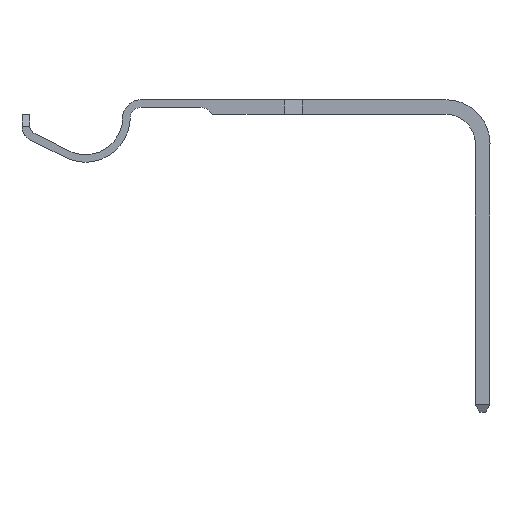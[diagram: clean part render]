
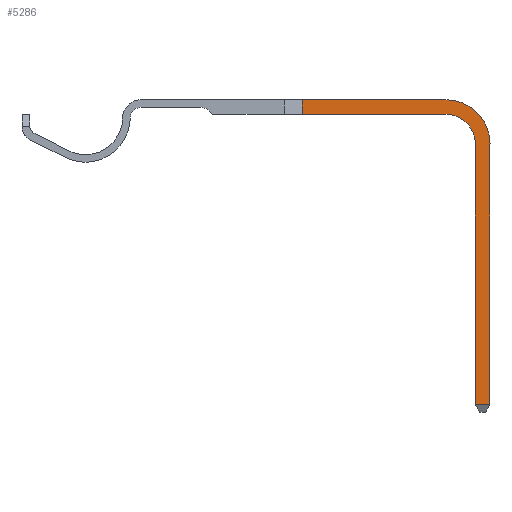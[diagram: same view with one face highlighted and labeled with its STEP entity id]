
A CAD part, left-side view. The second image highlights one B-rep face of the part: STEP entity #5286.
In plain terms, the highlighted face is planar.
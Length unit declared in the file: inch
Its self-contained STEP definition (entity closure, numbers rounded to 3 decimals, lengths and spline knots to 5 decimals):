
#418 = EDGE_CURVE ( 'NONE', #6218, #4069, #11643, .T. ) ;
#1639 = CARTESIAN_POINT ( 'NONE',  ( 0.85571, 0.0375, -0.0125 ) ) ;
#1671 = VECTOR ( 'NONE', #4748, 39.37008 ) ;
#1710 = CARTESIAN_POINT ( 'NONE',  ( 0.61115, 0.0375, -0.0125 ) ) ;
#2480 = VERTEX_POINT ( 'NONE', #5205 ) ;
#2566 = EDGE_LOOP ( 'NONE', ( #3363, #9571, #14567, #13523, #6890, #12255, #6935, #12614 ) ) ;
#2777 = CARTESIAN_POINT ( 'NONE',  ( 0.58021, 0.0125, -0.0125 ) ) ;
#2914 = CARTESIAN_POINT ( 'NONE',  ( 0.85571, 0.0875, -0.0125 ) ) ;
#2934 = DIRECTION ( 'NONE',  ( 0., 1., 0. ) ) ;
#3066 = VECTOR ( 'NONE', #7339, 39.37008 ) ;
#3363 = ORIENTED_EDGE ( 'NONE', *, *, #6491, .T. ) ;
#3424 = LINE ( 'NONE', #2777, #3066 ) ;
#3797 = EDGE_CURVE ( 'NONE', #11314, #6218, #3424, .T. ) ;
#4069 = VERTEX_POINT ( 'NONE', #1710 ) ;
#4230 = EDGE_CURVE ( 'NONE', #9827, #13113, #6945, .T. ) ;
#4748 = DIRECTION ( 'NONE',  ( 0., 1., 0. ) ) ;
#4835 = CARTESIAN_POINT ( 'NONE',  ( 0.93071, 0.532, -0.0125 ) ) ;
#5205 = CARTESIAN_POINT ( 'NONE',  ( 0.93071, 0.0875, -0.0125 ) ) ;
#5286 = ADVANCED_FACE ( 'NONE', ( #10109 ), #13745, .F. ) ;
#5459 = CARTESIAN_POINT ( 'NONE',  ( 0.61115, 0.0875, -0.0125 ) ) ;
#5632 = VECTOR ( 'NONE', #2934, 39.37008 ) ;
#5665 = CIRCLE ( 'NONE', #13672, 0.075 ) ;
#6218 = VERTEX_POINT ( 'NONE', #14298 ) ;
#6317 = LINE ( 'NONE', #8318, #11623 ) ;
#6491 = EDGE_CURVE ( 'NONE', #13113, #14999, #10647, .T. ) ;
#6619 = DIRECTION ( 'NONE',  ( 0., 0., -1. ) ) ;
#6890 = ORIENTED_EDGE ( 'NONE', *, *, #3797, .T. ) ;
#6935 = ORIENTED_EDGE ( 'NONE', *, *, #11959, .T. ) ;
#6945 = CIRCLE ( 'NONE', #12602, 0.05 ) ;
#7013 = CARTESIAN_POINT ( 'NONE',  ( 0.85571, 0.0125, -0.0125 ) ) ;
#7048 = DIRECTION ( 'NONE',  ( 1., 0., 0. ) ) ;
#7081 = CARTESIAN_POINT ( 'NONE',  ( 0.90571, 0.0875, -0.0125 ) ) ;
#7267 = LINE ( 'NONE', #7586, #10278 ) ;
#7339 = DIRECTION ( 'NONE',  ( -1., 0., 0. ) ) ;
#7586 = CARTESIAN_POINT ( 'NONE',  ( 0.93071, 0.0875, -0.0125 ) ) ;
#7869 = DIRECTION ( 'NONE',  ( 1., 0., 0. ) ) ;
#8145 = CARTESIAN_POINT ( 'NONE',  ( 0.58021, 0.0375, -0.0125 ) ) ;
#8220 = CARTESIAN_POINT ( 'NONE',  ( 0.90571, 0.532, -0.0125 ) ) ;
#8318 = CARTESIAN_POINT ( 'NONE',  ( 0.85571, 0.532, -0.0125 ) ) ;
#8716 = DIRECTION ( 'NONE',  ( 0., -1., 0. ) ) ;
#8880 = AXIS2_PLACEMENT_3D ( 'NONE', #2914, #10603, #7869 ) ;
#9465 = CARTESIAN_POINT ( 'NONE',  ( 0.85571, 0.0875, -0.0125 ) ) ;
#9571 = ORIENTED_EDGE ( 'NONE', *, *, #9652, .T. ) ;
#9652 = EDGE_CURVE ( 'NONE', #14999, #13234, #6317, .T. ) ;
#9827 = VERTEX_POINT ( 'NONE', #1639 ) ;
#10109 = FACE_OUTER_BOUND ( 'NONE', #2566, .T. ) ;
#10278 = VECTOR ( 'NONE', #8716, 39.37008 ) ;
#10305 = LINE ( 'NONE', #8145, #12647 ) ;
#10510 = DIRECTION ( 'NONE',  ( 1., 0., 0. ) ) ;
#10603 = DIRECTION ( 'NONE',  ( 0., 0., 1. ) ) ;
#10647 = LINE ( 'NONE', #7081, #1671 ) ;
#11177 = DIRECTION ( 'NONE',  ( 0., 0., 1. ) ) ;
#11314 = VERTEX_POINT ( 'NONE', #7013 ) ;
#11623 = VECTOR ( 'NONE', #12855, 39.37008 ) ;
#11643 = LINE ( 'NONE', #5459, #5632 ) ;
#11959 = EDGE_CURVE ( 'NONE', #4069, #9827, #10305, .T. ) ;
#12255 = ORIENTED_EDGE ( 'NONE', *, *, #418, .T. ) ;
#12602 = AXIS2_PLACEMENT_3D ( 'NONE', #9465, #11177, #10510 ) ;
#12611 = CARTESIAN_POINT ( 'NONE',  ( 0.90571, 0.0875, -0.0125 ) ) ;
#12614 = ORIENTED_EDGE ( 'NONE', *, *, #4230, .T. ) ;
#12647 = VECTOR ( 'NONE', #7048, 39.37008 ) ;
#12792 = EDGE_CURVE ( 'NONE', #13234, #2480, #7267, .T. ) ;
#12855 = DIRECTION ( 'NONE',  ( 1., 0., 0. ) ) ;
#13113 = VERTEX_POINT ( 'NONE', #12611 ) ;
#13234 = VERTEX_POINT ( 'NONE', #4835 ) ;
#13453 = CARTESIAN_POINT ( 'NONE',  ( 0.85571, 0.0875, -0.0125 ) ) ;
#13523 = ORIENTED_EDGE ( 'NONE', *, *, #13573, .T. ) ;
#13573 = EDGE_CURVE ( 'NONE', #2480, #11314, #5665, .T. ) ;
#13672 = AXIS2_PLACEMENT_3D ( 'NONE', #13453, #6619, #14611 ) ;
#13745 = PLANE ( 'NONE',  #8880 ) ;
#14298 = CARTESIAN_POINT ( 'NONE',  ( 0.61115, 0.0125, -0.0125 ) ) ;
#14567 = ORIENTED_EDGE ( 'NONE', *, *, #12792, .T. ) ;
#14611 = DIRECTION ( 'NONE',  ( 1., 0., 0. ) ) ;
#14999 = VERTEX_POINT ( 'NONE', #8220 ) ;
